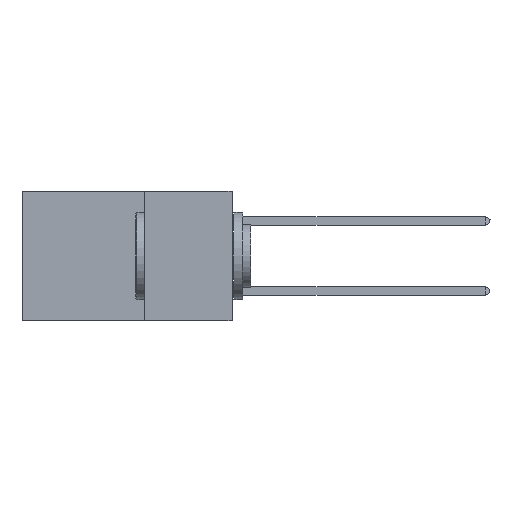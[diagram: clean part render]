
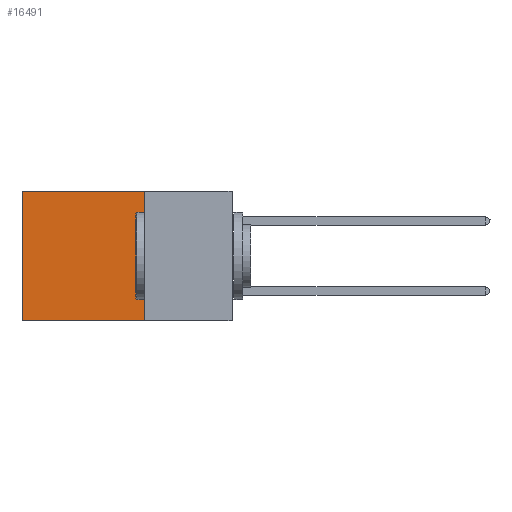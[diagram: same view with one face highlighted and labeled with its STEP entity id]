
A CAD part, left-side view. The second image highlights one B-rep face of the part: STEP entity #16491.
In plain terms, the highlighted planar face has unit normal (-1, 0, 0).
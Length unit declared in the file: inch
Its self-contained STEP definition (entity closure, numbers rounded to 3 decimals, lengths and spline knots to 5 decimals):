
#488 = ORIENTED_EDGE ( 'NONE', *, *, #26587, .F. ) ;
#1124 = VERTEX_POINT ( 'NONE', #23361 ) ;
#1219 = CARTESIAN_POINT ( 'NONE',  ( 0.2875, 0.25, -0.37 ) ) ;
#2389 = EDGE_CURVE ( 'NONE', #26019, #27068, #10673, .T. ) ;
#4666 = VECTOR ( 'NONE', #25311, 39.37008 ) ;
#4827 = PLANE ( 'NONE',  #22377 ) ;
#6589 = VERTEX_POINT ( 'NONE', #1219 ) ;
#6923 = LINE ( 'NONE', #31077, #23018 ) ;
#6974 = CARTESIAN_POINT ( 'NONE',  ( 0.2875, 0.25, 0. ) ) ;
#7461 = FACE_OUTER_BOUND ( 'NONE', #18338, .T. ) ;
#9534 = DIRECTION ( 'NONE',  ( 0., 1., 0. ) ) ;
#10673 = LINE ( 'NONE', #30208, #4666 ) ;
#10674 = VECTOR ( 'NONE', #11989, 39.37008 ) ;
#11889 = CARTESIAN_POINT ( 'NONE',  ( 0.2875, 0.25, 0. ) ) ;
#11989 = DIRECTION ( 'NONE',  ( 0., 0., -1. ) ) ;
#13472 = VECTOR ( 'NONE', #9534, 39.37008 ) ;
#13817 = CARTESIAN_POINT ( 'NONE',  ( 0.2875, 0.6, -0.37 ) ) ;
#14728 = EDGE_CURVE ( 'NONE', #1124, #26019, #27257, .T. ) ;
#15056 = DIRECTION ( 'NONE',  ( 0., 0., -1. ) ) ;
#16491 = ADVANCED_FACE ( 'NONE', ( #7461 ), #4827, .F. ) ;
#17371 = CARTESIAN_POINT ( 'NONE',  ( 0.2875, 0.6, 0. ) ) ;
#18338 = EDGE_LOOP ( 'NONE', ( #28159, #19892, #488, #23749 ) ) ;
#19892 = ORIENTED_EDGE ( 'NONE', *, *, #22749, .F. ) ;
#22311 = CARTESIAN_POINT ( 'NONE',  ( 0.2875, 0.25, 0. ) ) ;
#22377 = AXIS2_PLACEMENT_3D ( 'NONE', #22311, #29646, #15056 ) ;
#22749 = EDGE_CURVE ( 'NONE', #6589, #27068, #6923, .T. ) ;
#23018 = VECTOR ( 'NONE', #23850, 39.37008 ) ;
#23361 = CARTESIAN_POINT ( 'NONE',  ( 0.2875, 0.25, 0. ) ) ;
#23749 = ORIENTED_EDGE ( 'NONE', *, *, #14728, .T. ) ;
#23850 = DIRECTION ( 'NONE',  ( 0., 1., 0. ) ) ;
#25311 = DIRECTION ( 'NONE',  ( 0., 0., -1. ) ) ;
#26019 = VERTEX_POINT ( 'NONE', #17371 ) ;
#26587 = EDGE_CURVE ( 'NONE', #1124, #6589, #31787, .T. ) ;
#27068 = VERTEX_POINT ( 'NONE', #13817 ) ;
#27257 = LINE ( 'NONE', #6974, #13472 ) ;
#28159 = ORIENTED_EDGE ( 'NONE', *, *, #2389, .T. ) ;
#29646 = DIRECTION ( 'NONE',  ( 1., 0., 0. ) ) ;
#30208 = CARTESIAN_POINT ( 'NONE',  ( 0.2875, 0.6, 0. ) ) ;
#31077 = CARTESIAN_POINT ( 'NONE',  ( 0.2875, 0.25, -0.37 ) ) ;
#31787 = LINE ( 'NONE', #11889, #10674 ) ;
